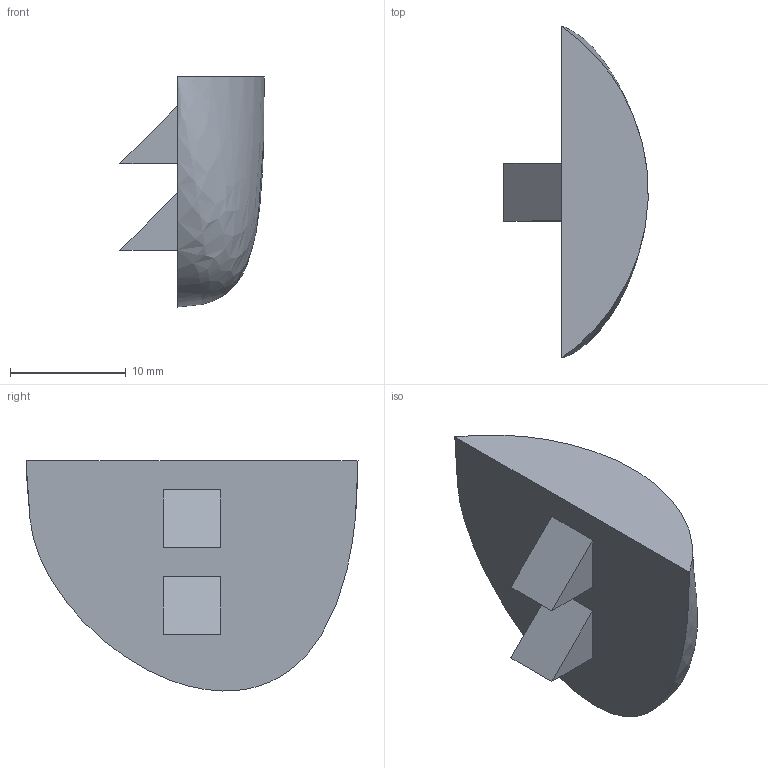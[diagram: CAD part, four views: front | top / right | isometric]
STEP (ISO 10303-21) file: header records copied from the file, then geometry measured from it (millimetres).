
FILE_DESCRIPTION (( 'STEP AP214' ), '1' );
FILE_NAME ('Barrel_Block_Left.step', '2015-01-13T04:29:55', ( '' ), ( '' ), 'SwSTEP 2.0', 'SolidWorks 2015', '' );
FILE_SCHEMA (( 'AUTOMOTIVE_DESIGN' ));
Length unit declared in the file: millimetre
Products named in the file (1): Barrel_Block_Left
Bounding box: 12.49 x 28.72 x 19.9 mm (x, y, z)
Volume: 2551.3 mm3; surface area: 1365 mm2
Topology: 1 solids, 1 shells, 11 faces, 24 edges, 15 vertices
Faces by surface type: plane 10, bspline 1
Entity records: 453 total; most frequent: CARTESIAN_POINT 193, ORIENTED_EDGE 44, DIRECTION 41, EDGE_CURVE 22, LINE 19, VECTOR 19, VERTEX_POINT 15, EDGE_LOOP 13
